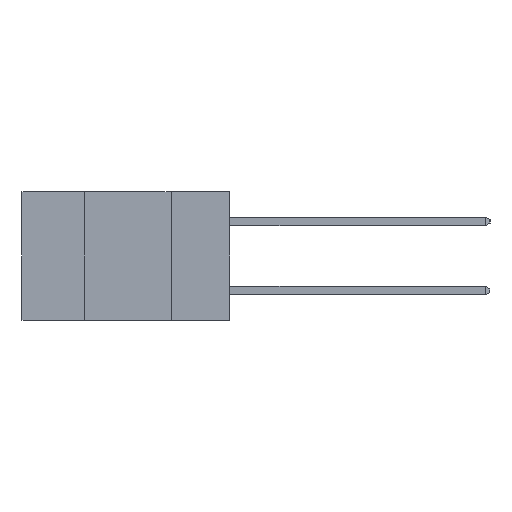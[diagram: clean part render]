
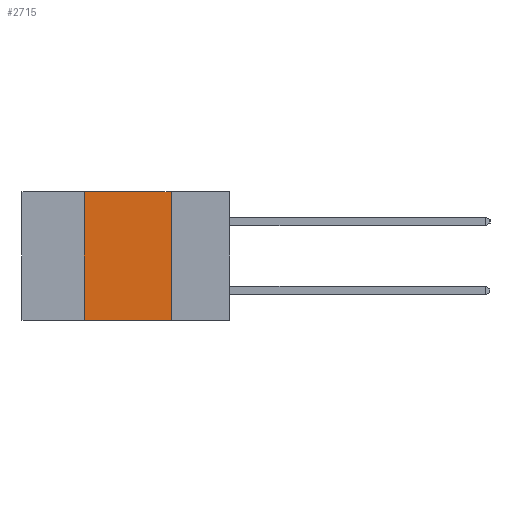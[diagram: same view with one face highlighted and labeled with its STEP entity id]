
A CAD part, left-side view. The second image highlights one B-rep face of the part: STEP entity #2715.
In plain terms, the highlighted planar face has unit normal (-1, 0, 0).
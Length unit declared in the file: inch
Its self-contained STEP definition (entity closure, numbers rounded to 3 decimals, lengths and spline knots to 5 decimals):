
#390 = VECTOR ( 'NONE', #2206, 39.37008 ) ;
#932 = VECTOR ( 'NONE', #8129, 39.37008 ) ;
#941 = ORIENTED_EDGE ( 'NONE', *, *, #4549, .F. ) ;
#1857 = VECTOR ( 'NONE', #5678, 39.37008 ) ;
#1884 = CARTESIAN_POINT ( 'NONE',  ( 0., 0.42, -0.37 ) ) ;
#2048 = VERTEX_POINT ( 'NONE', #9021 ) ;
#2206 = DIRECTION ( 'NONE',  ( 0., 0., -1. ) ) ;
#2619 = DIRECTION ( 'NONE',  ( 0., -1., 0. ) ) ;
#2715 = ADVANCED_FACE ( 'NONE', ( #12328 ), #7262, .F. ) ;
#2918 = CARTESIAN_POINT ( 'NONE',  ( 0., 0.42, 0. ) ) ;
#2976 = VERTEX_POINT ( 'NONE', #8114 ) ;
#3072 = EDGE_LOOP ( 'NONE', ( #5717, #6085, #941, #3722 ) ) ;
#3158 = EDGE_CURVE ( 'NONE', #8490, #10833, #4993, .T. ) ;
#3722 = ORIENTED_EDGE ( 'NONE', *, *, #3158, .T. ) ;
#4549 = EDGE_CURVE ( 'NONE', #8490, #2048, #8885, .T. ) ;
#4993 = LINE ( 'NONE', #10159, #1857 ) ;
#5678 = DIRECTION ( 'NONE',  ( 0., -1., 0. ) ) ;
#5717 = ORIENTED_EDGE ( 'NONE', *, *, #6617, .F. ) ;
#6085 = ORIENTED_EDGE ( 'NONE', *, *, #10227, .F. ) ;
#6104 = AXIS2_PLACEMENT_3D ( 'NONE', #8179, #8147, #10371 ) ;
#6617 = EDGE_CURVE ( 'NONE', #2976, #10833, #8678, .T. ) ;
#6679 = CARTESIAN_POINT ( 'NONE',  ( 0., 0.17, -0.37 ) ) ;
#7262 = PLANE ( 'NONE',  #6104 ) ;
#7636 = LINE ( 'NONE', #12629, #9975 ) ;
#8114 = CARTESIAN_POINT ( 'NONE',  ( 0., 0.17, 0. ) ) ;
#8129 = DIRECTION ( 'NONE',  ( 0., 0., 1. ) ) ;
#8147 = DIRECTION ( 'NONE',  ( 1., 0., 0. ) ) ;
#8179 = CARTESIAN_POINT ( 'NONE',  ( 0., 0.6, 0. ) ) ;
#8490 = VERTEX_POINT ( 'NONE', #1884 ) ;
#8678 = LINE ( 'NONE', #10370, #390 ) ;
#8885 = LINE ( 'NONE', #2918, #932 ) ;
#9021 = CARTESIAN_POINT ( 'NONE',  ( 0., 0.42, 0. ) ) ;
#9975 = VECTOR ( 'NONE', #2619, 39.37008 ) ;
#10159 = CARTESIAN_POINT ( 'NONE',  ( 0., 0.6, -0.37 ) ) ;
#10227 = EDGE_CURVE ( 'NONE', #2048, #2976, #7636, .T. ) ;
#10370 = CARTESIAN_POINT ( 'NONE',  ( 0., 0.17, 0. ) ) ;
#10371 = DIRECTION ( 'NONE',  ( 0., 0., -1. ) ) ;
#10833 = VERTEX_POINT ( 'NONE', #6679 ) ;
#12328 = FACE_OUTER_BOUND ( 'NONE', #3072, .T. ) ;
#12629 = CARTESIAN_POINT ( 'NONE',  ( 0., 0.6, 0. ) ) ;
